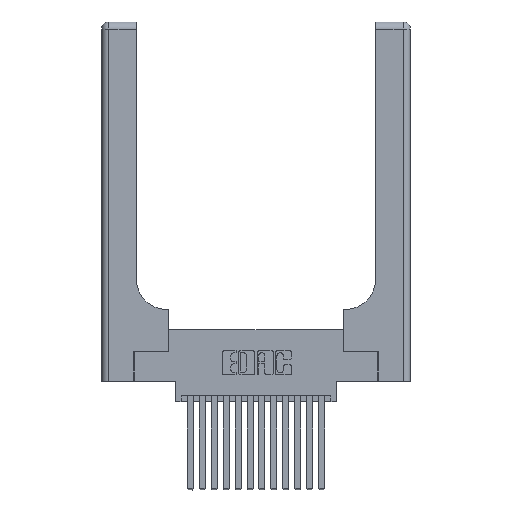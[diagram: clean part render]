
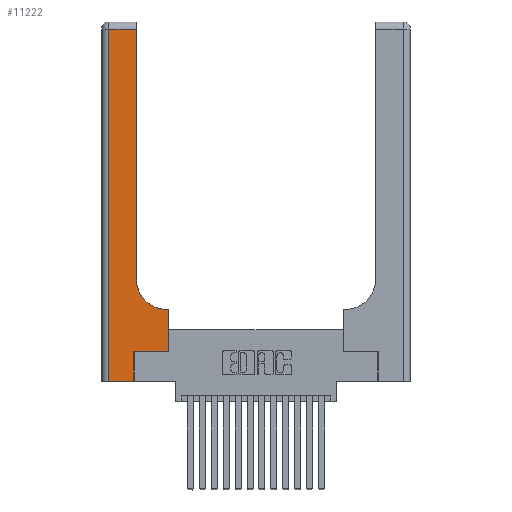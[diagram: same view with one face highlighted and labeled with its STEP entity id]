
A CAD part, top view. The second image highlights one B-rep face of the part: STEP entity #11222.
In plain terms, the highlighted planar face has unit normal (0, 0, 1).
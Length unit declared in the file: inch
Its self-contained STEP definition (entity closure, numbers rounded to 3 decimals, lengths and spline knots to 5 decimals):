
#92 = LINE ( 'NONE', #14813, #13796 ) ;
#413 = VERTEX_POINT ( 'NONE', #11865 ) ;
#432 = ORIENTED_EDGE ( 'NONE', *, *, #4881, .T. ) ;
#559 = FACE_OUTER_BOUND ( 'NONE', #15698, .T. ) ;
#570 = DIRECTION ( 'NONE',  ( 0., 0., -1. ) ) ;
#954 = CARTESIAN_POINT ( 'NONE',  ( 0.2915, 0.6, 0.37 ) ) ;
#1066 = VECTOR ( 'NONE', #15808, 39.37008 ) ;
#1449 = ORIENTED_EDGE ( 'NONE', *, *, #15570, .T. ) ;
#1462 = DIRECTION ( 'NONE',  ( -1., 0., 0. ) ) ;
#1519 = VERTEX_POINT ( 'NONE', #13469 ) ;
#1810 = ORIENTED_EDGE ( 'NONE', *, *, #10206, .T. ) ;
#1957 = LINE ( 'NONE', #954, #13409 ) ;
#2056 = ORIENTED_EDGE ( 'NONE', *, *, #6870, .T. ) ;
#2058 = CARTESIAN_POINT ( 'NONE',  ( 0.2915, 2.94, 0.37 ) ) ;
#2456 = CARTESIAN_POINT ( 'NONE',  ( 0.2915, 0.85, 0.37 ) ) ;
#2584 = CARTESIAN_POINT ( 'NONE',  ( 0.2915, 3., 0.37 ) ) ;
#2963 = DIRECTION ( 'NONE',  ( 0., 0., -1. ) ) ;
#3256 = ORIENTED_EDGE ( 'NONE', *, *, #11411, .T. ) ;
#3361 = CARTESIAN_POINT ( 'NONE',  ( 0.5415, 0.6, 0.37 ) ) ;
#3873 = CARTESIAN_POINT ( 'NONE',  ( 0.269, 0., 0.37 ) ) ;
#4346 = CARTESIAN_POINT ( 'NONE',  ( 0., 0., 0.37 ) ) ;
#4449 = CARTESIAN_POINT ( 'NONE',  ( 0.06, 0., 0.37 ) ) ;
#4686 = CIRCLE ( 'NONE', #13827, 0.25 ) ;
#4749 = VERTEX_POINT ( 'NONE', #2456 ) ;
#4773 = VECTOR ( 'NONE', #6978, 39.37008 ) ;
#4881 = EDGE_CURVE ( 'NONE', #6020, #1519, #7696, .T. ) ;
#4956 = VECTOR ( 'NONE', #17321, 39.37008 ) ;
#5178 = VERTEX_POINT ( 'NONE', #2058 ) ;
#5339 = ORIENTED_EDGE ( 'NONE', *, *, #8400, .T. ) ;
#5479 = LINE ( 'NONE', #2584, #4773 ) ;
#5558 = VECTOR ( 'NONE', #12210, 39.37008 ) ;
#6020 = VERTEX_POINT ( 'NONE', #3873 ) ;
#6424 = VECTOR ( 'NONE', #13826, 39.37008 ) ;
#6658 = VERTEX_POINT ( 'NONE', #4449 ) ;
#6870 = EDGE_CURVE ( 'NONE', #17665, #4749, #4686, .T. ) ;
#6978 = DIRECTION ( 'NONE',  ( 0., 1., 0. ) ) ;
#7013 = CARTESIAN_POINT ( 'NONE',  ( 0., 2.94, 0.37 ) ) ;
#7696 = LINE ( 'NONE', #9948, #4956 ) ;
#8400 = EDGE_CURVE ( 'NONE', #15409, #17665, #1957, .T. ) ;
#8506 = CARTESIAN_POINT ( 'NONE',  ( 0.269, 0.25, 0.37 ) ) ;
#8707 = LINE ( 'NONE', #4346, #1066 ) ;
#9111 = ORIENTED_EDGE ( 'NONE', *, *, #17967, .T. ) ;
#9338 = VERTEX_POINT ( 'NONE', #10588 ) ;
#9401 = CARTESIAN_POINT ( 'NONE',  ( 0.06, 3., 0.37 ) ) ;
#9948 = CARTESIAN_POINT ( 'NONE',  ( 0.269, 0., 0.37 ) ) ;
#10060 = AXIS2_PLACEMENT_3D ( 'NONE', #10196, #2963, #1462 ) ;
#10196 = CARTESIAN_POINT ( 'NONE',  ( 0., 3., 0.37 ) ) ;
#10206 = EDGE_CURVE ( 'NONE', #9338, #6658, #11870, .T. ) ;
#10588 = CARTESIAN_POINT ( 'NONE',  ( 0.06, 2.94, 0.37 ) ) ;
#11126 = VECTOR ( 'NONE', #14164, 39.37008 ) ;
#11204 = ORIENTED_EDGE ( 'NONE', *, *, #14404, .T. ) ;
#11222 = ADVANCED_FACE ( 'NONE', ( #559 ), #12885, .F. ) ;
#11411 = EDGE_CURVE ( 'NONE', #413, #15409, #92, .T. ) ;
#11591 = EDGE_CURVE ( 'NONE', #4749, #5178, #5479, .T. ) ;
#11865 = CARTESIAN_POINT ( 'NONE',  ( 0.5585, 0.25, 0.37 ) ) ;
#11870 = LINE ( 'NONE', #9401, #5558 ) ;
#11978 = CARTESIAN_POINT ( 'NONE',  ( 0.5585, 0.6, 0.37 ) ) ;
#12210 = DIRECTION ( 'NONE',  ( 0., -1., 0. ) ) ;
#12885 = PLANE ( 'NONE',  #10060 ) ;
#13409 = VECTOR ( 'NONE', #16754, 39.37008 ) ;
#13469 = CARTESIAN_POINT ( 'NONE',  ( 0.269, 0.25, 0.37 ) ) ;
#13559 = LINE ( 'NONE', #7013, #11126 ) ;
#13796 = VECTOR ( 'NONE', #16273, 39.37008 ) ;
#13826 = DIRECTION ( 'NONE',  ( 1., 0., 0. ) ) ;
#13827 = AXIS2_PLACEMENT_3D ( 'NONE', #15057, #570, #18015 ) ;
#14164 = DIRECTION ( 'NONE',  ( -1., 0., 0. ) ) ;
#14404 = EDGE_CURVE ( 'NONE', #1519, #413, #16991, .T. ) ;
#14813 = CARTESIAN_POINT ( 'NONE',  ( 0.5585, 0.25, 0.37 ) ) ;
#15057 = CARTESIAN_POINT ( 'NONE',  ( 0.5415, 0.85, 0.37 ) ) ;
#15409 = VERTEX_POINT ( 'NONE', #11978 ) ;
#15542 = ORIENTED_EDGE ( 'NONE', *, *, #11591, .T. ) ;
#15570 = EDGE_CURVE ( 'NONE', #5178, #9338, #13559, .T. ) ;
#15698 = EDGE_LOOP ( 'NONE', ( #15542, #1449, #1810, #9111, #432, #11204, #3256, #5339, #2056 ) ) ;
#15808 = DIRECTION ( 'NONE',  ( 1., 0., 0. ) ) ;
#16273 = DIRECTION ( 'NONE',  ( 0., 1., 0. ) ) ;
#16754 = DIRECTION ( 'NONE',  ( -1., 0., 0. ) ) ;
#16991 = LINE ( 'NONE', #8506, #6424 ) ;
#17321 = DIRECTION ( 'NONE',  ( 0., 1., 0. ) ) ;
#17665 = VERTEX_POINT ( 'NONE', #3361 ) ;
#17967 = EDGE_CURVE ( 'NONE', #6658, #6020, #8707, .T. ) ;
#18015 = DIRECTION ( 'NONE',  ( 1., 0., 0. ) ) ;
